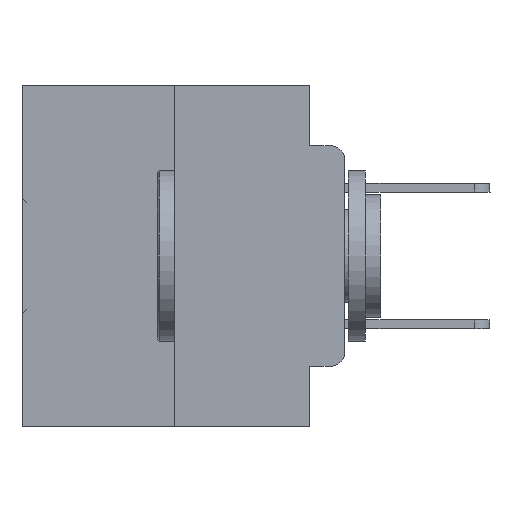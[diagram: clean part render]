
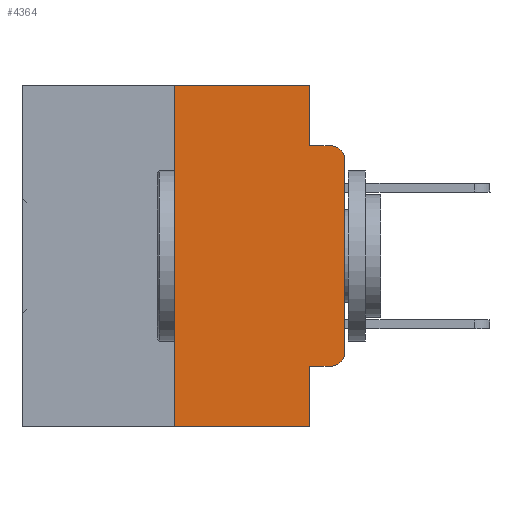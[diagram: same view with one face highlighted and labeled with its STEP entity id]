
A CAD part, left-side view. The second image highlights one B-rep face of the part: STEP entity #4364.
In plain terms, the highlighted planar face has unit normal (-1, 0, 0).
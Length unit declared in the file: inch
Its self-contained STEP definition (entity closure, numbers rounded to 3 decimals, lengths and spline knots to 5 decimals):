
#483 = CARTESIAN_POINT ( 'NONE',  ( 0., 0.473, 0. ) ) ;
#554 = VERTEX_POINT ( 'NONE', #17095 ) ;
#986 = ORIENTED_EDGE ( 'NONE', *, *, #4503, .T. ) ;
#2216 = EDGE_CURVE ( 'NONE', #28984, #33692, #27813, .T. ) ;
#2898 = LINE ( 'NONE', #24724, #16195 ) ;
#3487 = EDGE_CURVE ( 'NONE', #28984, #554, #12569, .T. ) ;
#3655 = EDGE_CURVE ( 'NONE', #33692, #29757, #24433, .T. ) ;
#4000 = ORIENTED_EDGE ( 'NONE', *, *, #3655, .T. ) ;
#4364 = ADVANCED_FACE ( 'NONE', ( #28252 ), #31474, .F. ) ;
#4503 = EDGE_CURVE ( 'NONE', #29757, #6571, #12665, .T. ) ;
#4749 = AXIS2_PLACEMENT_3D ( 'NONE', #34149, #28072, #14477 ) ;
#4987 = AXIS2_PLACEMENT_3D ( 'NONE', #10767, #18492, #7901 ) ;
#6307 = ORIENTED_EDGE ( 'NONE', *, *, #17863, .F. ) ;
#6571 = VERTEX_POINT ( 'NONE', #14575 ) ;
#6900 = EDGE_CURVE ( 'NONE', #28320, #26686, #19689, .T. ) ;
#7569 = DIRECTION ( 'NONE',  ( 0., 0., -1. ) ) ;
#7730 = LINE ( 'NONE', #30120, #19226 ) ;
#7901 = DIRECTION ( 'NONE',  ( 0., 0., -1. ) ) ;
#7992 = ORIENTED_EDGE ( 'NONE', *, *, #2216, .T. ) ;
#8814 = CARTESIAN_POINT ( 'NONE',  ( 0., 0.051, -0.4115 ) ) ;
#8971 = ORIENTED_EDGE ( 'NONE', *, *, #3487, .F. ) ;
#9770 = CARTESIAN_POINT ( 'NONE',  ( 0., 0.051, -0.0885 ) ) ;
#9836 = DIRECTION ( 'NONE',  ( 0., -1., 0. ) ) ;
#10708 = CARTESIAN_POINT ( 'NONE',  ( 0., 0., -0.3915 ) ) ;
#10767 = CARTESIAN_POINT ( 'NONE',  ( 0., 0.02, -0.3915 ) ) ;
#12241 = ORIENTED_EDGE ( 'NONE', *, *, #17494, .F. ) ;
#12478 = VECTOR ( 'NONE', #35113, 39.37008 ) ;
#12569 = LINE ( 'NONE', #19799, #17012 ) ;
#12665 = LINE ( 'NONE', #34315, #24793 ) ;
#12764 = EDGE_CURVE ( 'NONE', #28478, #28320, #2898, .T. ) ;
#13898 = EDGE_LOOP ( 'NONE', ( #986, #16776, #21506, #17474, #12241, #6307, #26710, #8971, #7992, #4000 ) ) ;
#14477 = DIRECTION ( 'NONE',  ( 0., 0., -1. ) ) ;
#14575 = CARTESIAN_POINT ( 'NONE',  ( 0., 0., -0.1085 ) ) ;
#14735 = VECTOR ( 'NONE', #30211, 39.37008 ) ;
#15933 = CARTESIAN_POINT ( 'NONE',  ( 0., 0.02, -0.0885 ) ) ;
#16061 = VECTOR ( 'NONE', #9836, 39.37008 ) ;
#16097 = CARTESIAN_POINT ( 'NONE',  ( 0., 0.25, -0.5 ) ) ;
#16195 = VECTOR ( 'NONE', #27417, 39.37008 ) ;
#16776 = ORIENTED_EDGE ( 'NONE', *, *, #24483, .T. ) ;
#17012 = VECTOR ( 'NONE', #30722, 39.37008 ) ;
#17095 = CARTESIAN_POINT ( 'NONE',  ( 0., 0.051, -0.5 ) ) ;
#17474 = ORIENTED_EDGE ( 'NONE', *, *, #12764, .F. ) ;
#17494 = EDGE_CURVE ( 'NONE', #31079, #28478, #33212, .T. ) ;
#17863 = EDGE_CURVE ( 'NONE', #31169, #31079, #7730, .T. ) ;
#17990 = DIRECTION ( 'NONE',  ( -1., 0., 0. ) ) ;
#18188 = AXIS2_PLACEMENT_3D ( 'NONE', #35129, #17990, #7569 ) ;
#18492 = DIRECTION ( 'NONE',  ( -1., 0., 0. ) ) ;
#19226 = VECTOR ( 'NONE', #29941, 39.37008 ) ;
#19689 = LINE ( 'NONE', #22345, #12478 ) ;
#19799 = CARTESIAN_POINT ( 'NONE',  ( 0., 0.051, 0. ) ) ;
#19899 = EDGE_CURVE ( 'NONE', #31169, #554, #32921, .T. ) ;
#20897 = DIRECTION ( 'NONE',  ( 0., 0., 1. ) ) ;
#21444 = CARTESIAN_POINT ( 'NONE',  ( 0., 0.25, 0. ) ) ;
#21506 = ORIENTED_EDGE ( 'NONE', *, *, #6900, .F. ) ;
#22345 = CARTESIAN_POINT ( 'NONE',  ( 0., 0.051, -0.0885 ) ) ;
#23364 = CARTESIAN_POINT ( 'NONE',  ( 0., 0.051, 0. ) ) ;
#24433 = CIRCLE ( 'NONE', #4987, 0.02 ) ;
#24483 = EDGE_CURVE ( 'NONE', #6571, #26686, #27316, .T. ) ;
#24562 = CARTESIAN_POINT ( 'NONE',  ( 0., 0.051, -0.4115 ) ) ;
#24724 = CARTESIAN_POINT ( 'NONE',  ( 0., 0.051, 0. ) ) ;
#24793 = VECTOR ( 'NONE', #20897, 39.37008 ) ;
#26686 = VERTEX_POINT ( 'NONE', #15933 ) ;
#26710 = ORIENTED_EDGE ( 'NONE', *, *, #19899, .T. ) ;
#27316 = CIRCLE ( 'NONE', #18188, 0.02 ) ;
#27417 = DIRECTION ( 'NONE',  ( 0., 0., -1. ) ) ;
#27813 = LINE ( 'NONE', #8814, #16061 ) ;
#28072 = DIRECTION ( 'NONE',  ( 1., 0., 0. ) ) ;
#28252 = FACE_OUTER_BOUND ( 'NONE', #13898, .T. ) ;
#28320 = VERTEX_POINT ( 'NONE', #9770 ) ;
#28478 = VERTEX_POINT ( 'NONE', #23364 ) ;
#28984 = VERTEX_POINT ( 'NONE', #24562 ) ;
#29391 = CARTESIAN_POINT ( 'NONE',  ( 0., 0.02, -0.4115 ) ) ;
#29757 = VERTEX_POINT ( 'NONE', #10708 ) ;
#29941 = DIRECTION ( 'NONE',  ( 0., 0., 1. ) ) ;
#30120 = CARTESIAN_POINT ( 'NONE',  ( 0., 0.25, 0. ) ) ;
#30211 = DIRECTION ( 'NONE',  ( 0., -1., 0. ) ) ;
#30722 = DIRECTION ( 'NONE',  ( 0., 0., -1. ) ) ;
#30797 = DIRECTION ( 'NONE',  ( 0., -1., 0. ) ) ;
#31079 = VERTEX_POINT ( 'NONE', #21444 ) ;
#31169 = VERTEX_POINT ( 'NONE', #16097 ) ;
#31474 = PLANE ( 'NONE',  #4749 ) ;
#32748 = CARTESIAN_POINT ( 'NONE',  ( 0., 0.473, -0.5 ) ) ;
#32921 = LINE ( 'NONE', #32748, #34827 ) ;
#33212 = LINE ( 'NONE', #483, #14735 ) ;
#33692 = VERTEX_POINT ( 'NONE', #29391 ) ;
#34149 = CARTESIAN_POINT ( 'NONE',  ( 0., 0.473, 0. ) ) ;
#34315 = CARTESIAN_POINT ( 'NONE',  ( 0., 0., 0. ) ) ;
#34827 = VECTOR ( 'NONE', #30797, 39.37008 ) ;
#35113 = DIRECTION ( 'NONE',  ( 0., -1., 0. ) ) ;
#35129 = CARTESIAN_POINT ( 'NONE',  ( 0., 0.02, -0.1085 ) ) ;
